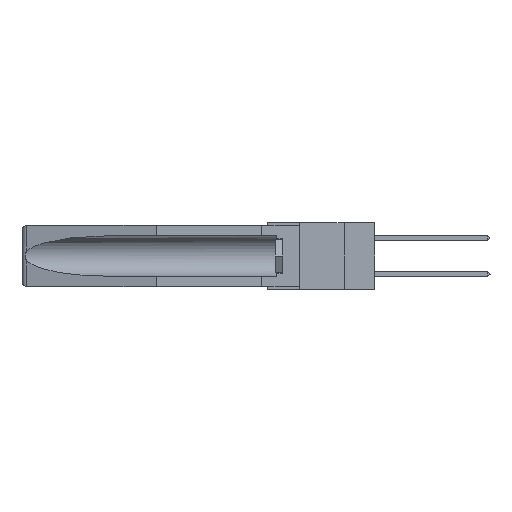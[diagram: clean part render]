
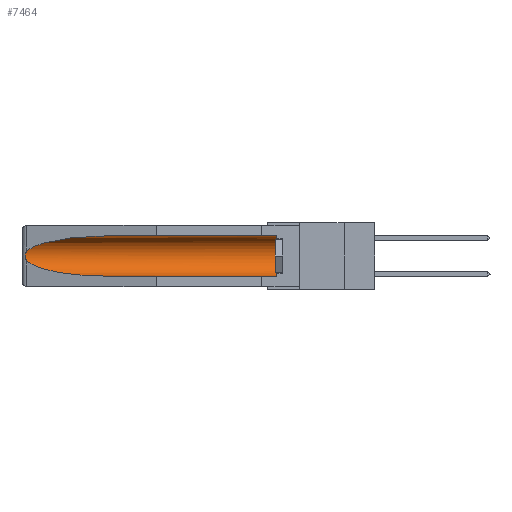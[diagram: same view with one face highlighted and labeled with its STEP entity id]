
A CAD part, left-side view. The second image highlights one B-rep face of the part: STEP entity #7464.
In plain terms, the highlighted cylindrical face has radius 2.857 mm (diameter 5.715 mm), a partial arc.
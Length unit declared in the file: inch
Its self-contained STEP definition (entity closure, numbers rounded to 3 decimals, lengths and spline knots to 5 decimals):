
#1312 = CARTESIAN_POINT ( 'NONE',  ( 0.2675, 1.53308, -0.17534 ) ) ;
#1351 = VERTEX_POINT ( 'NONE', #3468 ) ;
#1794 = DIRECTION ( 'NONE',  ( 0., 1., 0. ) ) ;
#1850 = DIRECTION ( 'NONE',  ( 0., 1., 0. ) ) ;
#1896 = VECTOR ( 'NONE', #1850, 39.37008 ) ;
#3155 = EDGE_LOOP ( 'NONE', ( #24230, #27062, #17797, #25729, #4746, #19429 ) ) ;
#3468 = CARTESIAN_POINT ( 'NONE',  ( 0.26537, 1.52718, -0.19328 ) ) ;
#4392 = LINE ( 'NONE', #25712, #1896 ) ;
#4664 = CARTESIAN_POINT ( 'NONE',  ( 0.155, 1.07973, -0.284 ) ) ;
#4746 = ORIENTED_EDGE ( 'NONE', *, *, #22708, .T. ) ;
#4971 = CARTESIAN_POINT ( 'NONE',  ( 0.155, 1.07973, -0.059 ) ) ;
#6235 = EDGE_CURVE ( 'NONE', #14431, #1351, #10878, .T. ) ;
#6294 = CARTESIAN_POINT ( 'NONE',  ( 0.2673, 1.5327, -0.16383 ) ) ;
#7137 = VERTEX_POINT ( 'NONE', #4971 ) ;
#7464 = ADVANCED_FACE ( 'NONE', ( #21779 ), #7627, .F. ) ;
#7482 = CARTESIAN_POINT ( 'NONE',  ( 0.155, -0.30754, -0.284 ) ) ;
#7627 = CYLINDRICAL_SURFACE ( 'NONE', #8050, 0.1125 ) ;
#8050 = AXIS2_PLACEMENT_3D ( 'NONE', #30245, #22284, #30136 ) ;
#9471 = CARTESIAN_POINT ( 'NONE',  ( 0.155, 1.07973, -0.284 ) ) ;
#9776 = CARTESIAN_POINT ( 'NONE',  ( 0.26537, 1.52718, -0.19328 ) ) ;
#10268 = DIRECTION ( 'NONE',  ( 0., 0., 1. ) ) ;
#10878 = B_SPLINE_CURVE_WITH_KNOTS ( 'NONE', 3,
 ( #11886, #30199, #27962, #6294, #14311, #1312, #11766, #22350, #33103, #33224 ),
 .UNSPECIFIED., .F., .F.,
 ( 4, 2, 2, 2, 4 ),
 ( 0., 0.00029, 0.00058, 0.00087, 0.00117 ),
 .UNSPECIFIED. ) ;
#11140 = CARTESIAN_POINT ( 'NONE',  ( 0.155, 0.126, -0.059 ) ) ;
#11766 = CARTESIAN_POINT ( 'NONE',  ( 0.2673, 1.53269, -0.17917 ) ) ;
#11886 = CARTESIAN_POINT ( 'NONE',  ( 0.26537, 1.52718, -0.14972 ) ) ;
#14311 = CARTESIAN_POINT ( 'NONE',  ( 0.2675, 1.53308, -0.16763 ) ) ;
#14431 = VERTEX_POINT ( 'NONE', #31864 ) ;
#15219 = CARTESIAN_POINT ( 'NONE',  ( 0.25451, 1.48313, -0.24835 ) ) ;
#15443 = CARTESIAN_POINT ( 'NONE',  ( 0.26537, 1.52718, -0.14972 ) ) ;
#16539 = CIRCLE ( 'NONE', #21180, 0.1125 ) ;
#16718 = VERTEX_POINT ( 'NONE', #20559 ) ;
#17047 =( BOUNDED_CURVE ( )  B_SPLINE_CURVE ( 3, ( #20457, #23138, #26290, #15443 ),
 .UNSPECIFIED., .F., .F. ) 
 B_SPLINE_CURVE_WITH_KNOTS ( ( 4, 4 ),
 ( 4.71239, 6.08839 ),
 .UNSPECIFIED. ) 
 CURVE ( )  GEOMETRIC_REPRESENTATION_ITEM ( )  RATIONAL_B_SPLINE_CURVE ( ( 1., 0.848, 0.848, 1. ) ) 
 REPRESENTATION_ITEM ( '' )  );
#17273 = VERTEX_POINT ( 'NONE', #9471 ) ;
#17797 = ORIENTED_EDGE ( 'NONE', *, *, #30207, .T. ) ;
#18502 = LINE ( 'NONE', #7482, #22655 ) ;
#18627 = EDGE_CURVE ( 'NONE', #34114, #7137, #4392, .T. ) ;
#19429 = ORIENTED_EDGE ( 'NONE', *, *, #18627, .T. ) ;
#20457 = CARTESIAN_POINT ( 'NONE',  ( 0.155, 1.07973, -0.059 ) ) ;
#20559 = CARTESIAN_POINT ( 'NONE',  ( 0.155, 0.126, -0.284 ) ) ;
#20615 = DIRECTION ( 'NONE',  ( 0., -1., 0. ) ) ;
#21180 = AXIS2_PLACEMENT_3D ( 'NONE', #33947, #20615, #10268 ) ;
#21779 = FACE_OUTER_BOUND ( 'NONE', #3155, .T. ) ;
#22284 = DIRECTION ( 'NONE',  ( 0., 1., 0. ) ) ;
#22350 = CARTESIAN_POINT ( 'NONE',  ( 0.26655, 1.53094, -0.18657 ) ) ;
#22655 = VECTOR ( 'NONE', #1794, 39.37008 ) ;
#22708 = EDGE_CURVE ( 'NONE', #16718, #34114, #16539, .T. ) ;
#23138 = CARTESIAN_POINT ( 'NONE',  ( 0.21114, 1.30732, -0.059 ) ) ;
#23162 = CARTESIAN_POINT ( 'NONE',  ( 0.21114, 1.30732, -0.284 ) ) ;
#24230 = ORIENTED_EDGE ( 'NONE', *, *, #27150, .T. ) ;
#24563 = EDGE_CURVE ( 'NONE', #16718, #17273, #18502, .T. ) ;
#25712 = CARTESIAN_POINT ( 'NONE',  ( 0.155, -0.30754, -0.059 ) ) ;
#25729 = ORIENTED_EDGE ( 'NONE', *, *, #24563, .F. ) ;
#26290 = CARTESIAN_POINT ( 'NONE',  ( 0.25451, 1.48313, -0.09465 ) ) ;
#27062 = ORIENTED_EDGE ( 'NONE', *, *, #6235, .T. ) ;
#27150 = EDGE_CURVE ( 'NONE', #7137, #14431, #17047, .T. ) ;
#27962 = CARTESIAN_POINT ( 'NONE',  ( 0.26654, 1.53092, -0.15636 ) ) ;
#30136 = DIRECTION ( 'NONE',  ( 0., 0., 1. ) ) ;
#30199 = CARTESIAN_POINT ( 'NONE',  ( 0.26597, 1.52961, -0.15275 ) ) ;
#30207 = EDGE_CURVE ( 'NONE', #1351, #17273, #33099, .T. ) ;
#30245 = CARTESIAN_POINT ( 'NONE',  ( 0.155, -0.30754, -0.1715 ) ) ;
#31864 = CARTESIAN_POINT ( 'NONE',  ( 0.26537, 1.52718, -0.14972 ) ) ;
#33099 =( BOUNDED_CURVE ( )  B_SPLINE_CURVE ( 3, ( #9776, #15219, #23162, #4664 ),
 .UNSPECIFIED., .F., .F. ) 
 B_SPLINE_CURVE_WITH_KNOTS ( ( 4, 4 ),
 ( 0.1948, 1.5708 ),
 .UNSPECIFIED. ) 
 CURVE ( )  GEOMETRIC_REPRESENTATION_ITEM ( )  RATIONAL_B_SPLINE_CURVE ( ( 1., 0.848, 0.848, 1. ) ) 
 REPRESENTATION_ITEM ( '' )  );
#33103 = CARTESIAN_POINT ( 'NONE',  ( 0.26597, 1.5296, -0.19026 ) ) ;
#33224 = CARTESIAN_POINT ( 'NONE',  ( 0.26537, 1.52718, -0.19328 ) ) ;
#33947 = CARTESIAN_POINT ( 'NONE',  ( 0.155, 0.126, -0.1715 ) ) ;
#34114 = VERTEX_POINT ( 'NONE', #11140 ) ;
